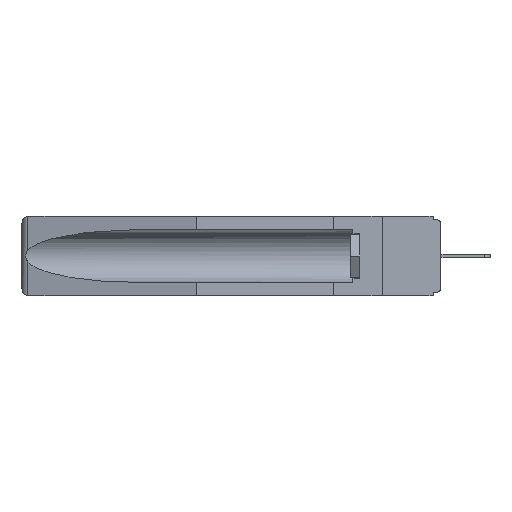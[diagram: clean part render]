
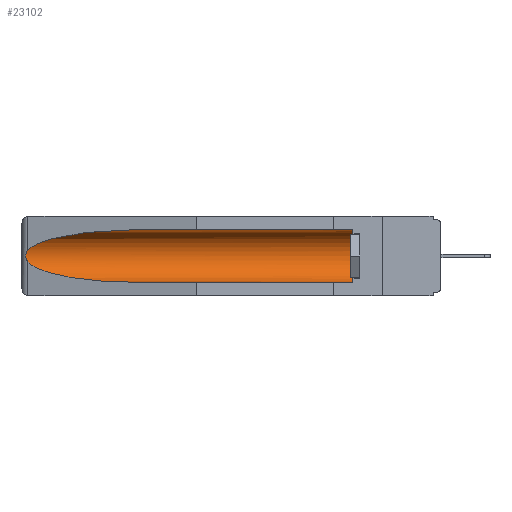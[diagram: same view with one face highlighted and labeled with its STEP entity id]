
A CAD part, left-side view. The second image highlights one B-rep face of the part: STEP entity #23102.
In plain terms, the highlighted cylindrical face has radius 2.857 mm (diameter 5.715 mm), a partial arc.
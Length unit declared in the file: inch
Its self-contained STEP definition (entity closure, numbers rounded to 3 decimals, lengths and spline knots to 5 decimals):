
#588 = CARTESIAN_POINT ( 'NONE',  ( 0.155, 1.07973, -0.059 ) ) ;
#706 = ORIENTED_EDGE ( 'NONE', *, *, #21544, .T. ) ;
#1766 = CARTESIAN_POINT ( 'NONE',  ( 0.26655, 1.53094, -0.18657 ) ) ;
#1988 = CARTESIAN_POINT ( 'NONE',  ( 0.155, 1.07973, -0.284 ) ) ;
#2285 = CARTESIAN_POINT ( 'NONE',  ( 0.155, 0.126, -0.1715 ) ) ;
#4197 = VERTEX_POINT ( 'NONE', #27701 ) ;
#4938 = ORIENTED_EDGE ( 'NONE', *, *, #7087, .T. ) ;
#5566 = CARTESIAN_POINT ( 'NONE',  ( 0.2675, 1.53308, -0.16763 ) ) ;
#5646 = AXIS2_PLACEMENT_3D ( 'NONE', #6678, #23934, #10909 ) ;
#6619 = EDGE_CURVE ( 'NONE', #10030, #4197, #16907, .T. ) ;
#6678 = CARTESIAN_POINT ( 'NONE',  ( 0.155, -0.30754, -0.1715 ) ) ;
#6808 = DIRECTION ( 'NONE',  ( 0., -1., 0. ) ) ;
#7087 = EDGE_CURVE ( 'NONE', #11227, #20112, #14043, .T. ) ;
#7670 = VECTOR ( 'NONE', #12108, 39.37008 ) ;
#7697 = CARTESIAN_POINT ( 'NONE',  ( 0.2673, 1.5327, -0.16383 ) ) ;
#7833 = CARTESIAN_POINT ( 'NONE',  ( 0.2673, 1.53269, -0.17917 ) ) ;
#9957 = CARTESIAN_POINT ( 'NONE',  ( 0.26597, 1.5296, -0.19026 ) ) ;
#10030 = VERTEX_POINT ( 'NONE', #10095 ) ;
#10095 = CARTESIAN_POINT ( 'NONE',  ( 0.155, 0.126, -0.284 ) ) ;
#10367 = CARTESIAN_POINT ( 'NONE',  ( 0.26537, 1.52718, -0.14972 ) ) ;
#10909 = DIRECTION ( 'NONE',  ( 0., 0., 1. ) ) ;
#11043 = CYLINDRICAL_SURFACE ( 'NONE', #5646, 0.1125 ) ;
#11144 = CARTESIAN_POINT ( 'NONE',  ( 0.25451, 1.48313, -0.24835 ) ) ;
#11227 = VERTEX_POINT ( 'NONE', #27215 ) ;
#11775 = LINE ( 'NONE', #22537, #11959 ) ;
#11804 = EDGE_CURVE ( 'NONE', #10030, #21439, #27188, .T. ) ;
#11959 = VECTOR ( 'NONE', #16031, 39.37008 ) ;
#12011 = EDGE_CURVE ( 'NONE', #21005, #11227, #26306, .T. ) ;
#12108 = DIRECTION ( 'NONE',  ( 0., 1., 0. ) ) ;
#12427 = ORIENTED_EDGE ( 'NONE', *, *, #6619, .F. ) ;
#12555 = ORIENTED_EDGE ( 'NONE', *, *, #22319, .T. ) ;
#12910 =( BOUNDED_CURVE ( )  B_SPLINE_CURVE ( 3, ( #13263, #11144, #25730, #1988 ),
 .UNSPECIFIED., .F., .F. ) 
 B_SPLINE_CURVE_WITH_KNOTS ( ( 4, 4 ),
 ( 0.1948, 1.5708 ),
 .UNSPECIFIED. ) 
 CURVE ( )  GEOMETRIC_REPRESENTATION_ITEM ( )  RATIONAL_B_SPLINE_CURVE ( ( 1., 0.848, 0.848, 1. ) ) 
 REPRESENTATION_ITEM ( '' )  );
#13089 = CARTESIAN_POINT ( 'NONE',  ( 0.155, 1.07973, -0.059 ) ) ;
#13263 = CARTESIAN_POINT ( 'NONE',  ( 0.26537, 1.52718, -0.19328 ) ) ;
#13589 = CARTESIAN_POINT ( 'NONE',  ( 0.26537, 1.52718, -0.14972 ) ) ;
#14043 = B_SPLINE_CURVE_WITH_KNOTS ( 'NONE', 3,
 ( #10367, #27063, #22822, #7697, #5566, #14743, #7833, #1766, #9957, #18574 ),
 .UNSPECIFIED., .F., .F.,
 ( 4, 2, 2, 2, 4 ),
 ( 0., 0.00029, 0.00058, 0.00087, 0.00117 ),
 .UNSPECIFIED. ) ;
#14528 = EDGE_LOOP ( 'NONE', ( #22910, #4938, #12555, #12427, #18233, #706 ) ) ;
#14743 = CARTESIAN_POINT ( 'NONE',  ( 0.2675, 1.53308, -0.17534 ) ) ;
#16031 = DIRECTION ( 'NONE',  ( 0., 1., 0. ) ) ;
#16907 = LINE ( 'NONE', #24983, #7670 ) ;
#17276 = CARTESIAN_POINT ( 'NONE',  ( 0.26537, 1.52718, -0.19328 ) ) ;
#18233 = ORIENTED_EDGE ( 'NONE', *, *, #11804, .T. ) ;
#18574 = CARTESIAN_POINT ( 'NONE',  ( 0.26537, 1.52718, -0.19328 ) ) ;
#19986 = CARTESIAN_POINT ( 'NONE',  ( 0.155, 0.126, -0.059 ) ) ;
#20112 = VERTEX_POINT ( 'NONE', #17276 ) ;
#21005 = VERTEX_POINT ( 'NONE', #13089 ) ;
#21439 = VERTEX_POINT ( 'NONE', #19986 ) ;
#21503 = DIRECTION ( 'NONE',  ( 0., 0., 1. ) ) ;
#21518 = FACE_OUTER_BOUND ( 'NONE', #14528, .T. ) ;
#21544 = EDGE_CURVE ( 'NONE', #21439, #21005, #11775, .T. ) ;
#22228 = AXIS2_PLACEMENT_3D ( 'NONE', #2285, #6808, #21503 ) ;
#22319 = EDGE_CURVE ( 'NONE', #20112, #4197, #12910, .T. ) ;
#22537 = CARTESIAN_POINT ( 'NONE',  ( 0.155, -0.30754, -0.059 ) ) ;
#22822 = CARTESIAN_POINT ( 'NONE',  ( 0.26654, 1.53092, -0.15636 ) ) ;
#22910 = ORIENTED_EDGE ( 'NONE', *, *, #12011, .T. ) ;
#23102 = ADVANCED_FACE ( 'NONE', ( #21518 ), #11043, .F. ) ;
#23934 = DIRECTION ( 'NONE',  ( 0., 1., 0. ) ) ;
#24332 = CARTESIAN_POINT ( 'NONE',  ( 0.25451, 1.48313, -0.09465 ) ) ;
#24983 = CARTESIAN_POINT ( 'NONE',  ( 0.155, -0.30754, -0.284 ) ) ;
#25730 = CARTESIAN_POINT ( 'NONE',  ( 0.21114, 1.30732, -0.284 ) ) ;
#26306 =( BOUNDED_CURVE ( )  B_SPLINE_CURVE ( 3, ( #588, #26444, #24332, #13589 ),
 .UNSPECIFIED., .F., .F. ) 
 B_SPLINE_CURVE_WITH_KNOTS ( ( 4, 4 ),
 ( 4.71239, 6.08839 ),
 .UNSPECIFIED. ) 
 CURVE ( )  GEOMETRIC_REPRESENTATION_ITEM ( )  RATIONAL_B_SPLINE_CURVE ( ( 1., 0.848, 0.848, 1. ) ) 
 REPRESENTATION_ITEM ( '' )  );
#26444 = CARTESIAN_POINT ( 'NONE',  ( 0.21114, 1.30732, -0.059 ) ) ;
#27063 = CARTESIAN_POINT ( 'NONE',  ( 0.26597, 1.52961, -0.15275 ) ) ;
#27188 = CIRCLE ( 'NONE', #22228, 0.1125 ) ;
#27215 = CARTESIAN_POINT ( 'NONE',  ( 0.26537, 1.52718, -0.14972 ) ) ;
#27701 = CARTESIAN_POINT ( 'NONE',  ( 0.155, 1.07973, -0.284 ) ) ;
